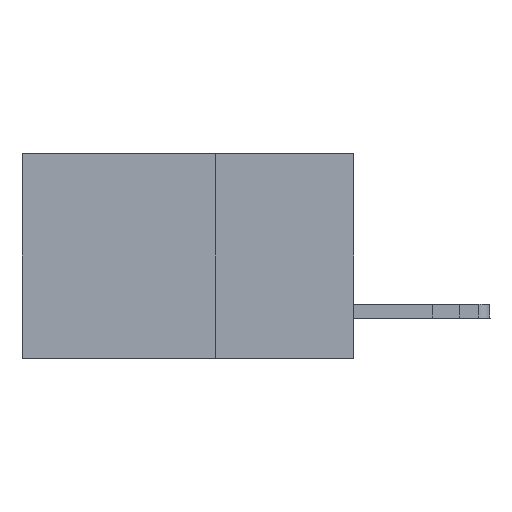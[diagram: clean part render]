
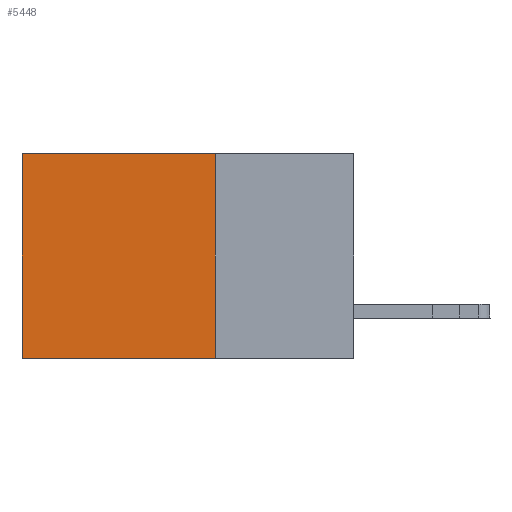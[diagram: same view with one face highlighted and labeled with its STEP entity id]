
A CAD part, left-side view. The second image highlights one B-rep face of the part: STEP entity #5448.
In plain terms, the highlighted planar face has unit normal (-1, 0, 0).
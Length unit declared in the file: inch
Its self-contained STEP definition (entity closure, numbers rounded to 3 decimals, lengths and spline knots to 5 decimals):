
#74 = VERTEX_POINT ( 'NONE', #315 ) ;
#315 = CARTESIAN_POINT ( 'NONE',  ( 0.2875, 0.25, 0. ) ) ;
#799 = VERTEX_POINT ( 'NONE', #2156 ) ;
#1670 = VERTEX_POINT ( 'NONE', #15325 ) ;
#2156 = CARTESIAN_POINT ( 'NONE',  ( 0.2875, 0.25, -0.37 ) ) ;
#3555 = LINE ( 'NONE', #17758, #15529 ) ;
#3728 = ORIENTED_EDGE ( 'NONE', *, *, #25421, .T. ) ;
#4038 = ORIENTED_EDGE ( 'NONE', *, *, #16267, .F. ) ;
#4308 = EDGE_CURVE ( 'NONE', #74, #1670, #14411, .T. ) ;
#4443 = EDGE_CURVE ( 'NONE', #74, #799, #22690, .T. ) ;
#5034 = FACE_OUTER_BOUND ( 'NONE', #14335, .T. ) ;
#5448 = ADVANCED_FACE ( 'NONE', ( #5034 ), #20485, .F. ) ;
#6742 = CARTESIAN_POINT ( 'NONE',  ( 0.2875, 0.25, 0. ) ) ;
#7783 = LINE ( 'NONE', #20478, #19746 ) ;
#7856 = CARTESIAN_POINT ( 'NONE',  ( 0.2875, 0.6, -0.37 ) ) ;
#10969 = VERTEX_POINT ( 'NONE', #7856 ) ;
#10983 = CARTESIAN_POINT ( 'NONE',  ( 0.2875, 0.25, 0. ) ) ;
#11160 = CARTESIAN_POINT ( 'NONE',  ( 0.2875, 0.25, 0. ) ) ;
#14335 = EDGE_LOOP ( 'NONE', ( #3728, #4038, #26766, #26374 ) ) ;
#14411 = LINE ( 'NONE', #11160, #20041 ) ;
#15325 = CARTESIAN_POINT ( 'NONE',  ( 0.2875, 0.6, 0. ) ) ;
#15529 = VECTOR ( 'NONE', #22648, 39.37008 ) ;
#15748 = DIRECTION ( 'NONE',  ( 0., 0., -1. ) ) ;
#16267 = EDGE_CURVE ( 'NONE', #799, #10969, #3555, .T. ) ;
#17758 = CARTESIAN_POINT ( 'NONE',  ( 0.2875, 0.25, -0.37 ) ) ;
#18739 = DIRECTION ( 'NONE',  ( 0., 0., -1. ) ) ;
#19746 = VECTOR ( 'NONE', #22912, 39.37008 ) ;
#20041 = VECTOR ( 'NONE', #27866, 39.37008 ) ;
#20478 = CARTESIAN_POINT ( 'NONE',  ( 0.2875, 0.6, 0. ) ) ;
#20485 = PLANE ( 'NONE',  #27222 ) ;
#21933 = VECTOR ( 'NONE', #18739, 39.37008 ) ;
#22648 = DIRECTION ( 'NONE',  ( 0., 1., 0. ) ) ;
#22690 = LINE ( 'NONE', #6742, #21933 ) ;
#22912 = DIRECTION ( 'NONE',  ( 0., 0., -1. ) ) ;
#25421 = EDGE_CURVE ( 'NONE', #1670, #10969, #7783, .T. ) ;
#26374 = ORIENTED_EDGE ( 'NONE', *, *, #4308, .T. ) ;
#26766 = ORIENTED_EDGE ( 'NONE', *, *, #4443, .F. ) ;
#27222 = AXIS2_PLACEMENT_3D ( 'NONE', #10983, #30030, #15748 ) ;
#27866 = DIRECTION ( 'NONE',  ( 0., 1., 0. ) ) ;
#30030 = DIRECTION ( 'NONE',  ( 1., 0., 0. ) ) ;
